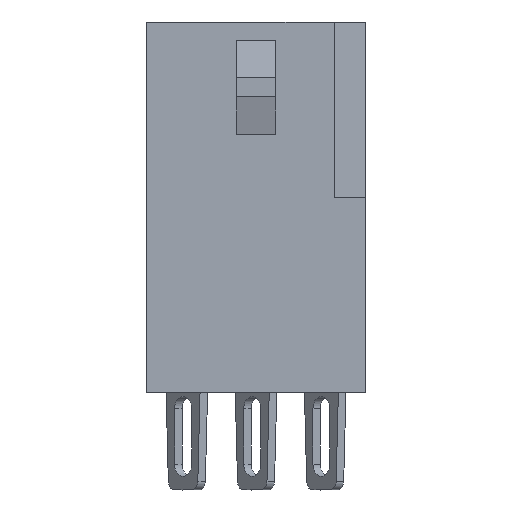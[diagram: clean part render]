
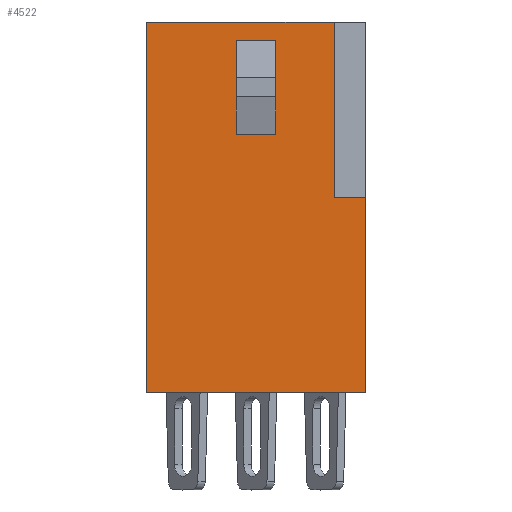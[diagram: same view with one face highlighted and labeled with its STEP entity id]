
A CAD part, top view. The second image highlights one B-rep face of the part: STEP entity #4522.
In plain terms, the highlighted planar face has unit normal (0, 0, 1).
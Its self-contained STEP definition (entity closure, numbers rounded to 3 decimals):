
#67 = EDGE_CURVE ( 'NONE', #673, #4810, #5719, .T. ) ;
#171 = LINE ( 'NONE', #1245, #2292 ) ;
#212 = CARTESIAN_POINT ( 'NONE',  ( 5.105, 8.991, 2.54 ) ) ;
#355 = CARTESIAN_POINT ( 'NONE',  ( 5.105, 8.992, 2.54 ) ) ;
#487 = ORIENTED_EDGE ( 'NONE', *, *, #4696, .T. ) ;
#583 = LINE ( 'NONE', #5169, #4838 ) ;
#605 = LINE ( 'NONE', #882, #5481 ) ;
#640 = ORIENTED_EDGE ( 'NONE', *, *, #2614, .F. ) ;
#652 = DIRECTION ( 'NONE',  ( 0., -1., 0. ) ) ;
#673 = VERTEX_POINT ( 'NONE', #4118 ) ;
#882 = CARTESIAN_POINT ( 'NONE',  ( -2.324, 10.033, 2.54 ) ) ;
#1026 = DIRECTION ( 'NONE',  ( -1., 0., 0. ) ) ;
#1198 = DIRECTION ( 'NONE',  ( -1., 0., 0. ) ) ;
#1245 = CARTESIAN_POINT ( 'NONE',  ( 7.339, 8.991, 2.54 ) ) ;
#1329 = CARTESIAN_POINT ( 'NONE',  ( 5.105, 3.608, 2.54 ) ) ;
#1357 = EDGE_CURVE ( 'NONE', #5795, #673, #6116, .T. ) ;
#1417 = LINE ( 'NONE', #4342, #2346 ) ;
#1470 = ORIENTED_EDGE ( 'NONE', *, *, #4973, .F. ) ;
#1475 = DIRECTION ( 'NONE',  ( 0., -1., 0. ) ) ;
#1613 = CARTESIAN_POINT ( 'NONE',  ( 8.445, 10.033, 2.54 ) ) ;
#1669 = VECTOR ( 'NONE', #5410, 1000. ) ;
#1874 = EDGE_CURVE ( 'NONE', #5945, #5450, #4713, .T. ) ;
#1972 = EDGE_CURVE ( 'NONE', #5797, #5795, #605, .T. ) ;
#2006 = CARTESIAN_POINT ( 'NONE',  ( -2.324, 0., 2.54 ) ) ;
#2188 = EDGE_CURVE ( 'NONE', #5945, #6157, #3814, .T. ) ;
#2202 = VERTEX_POINT ( 'NONE', #5382 ) ;
#2204 = DIRECTION ( 'NONE',  ( 1., 0., 0. ) ) ;
#2280 = VECTOR ( 'NONE', #5660, 1000. ) ;
#2292 = VECTOR ( 'NONE', #1198, 1000. ) ;
#2303 = DIRECTION ( 'NONE',  ( 1., 0., 0. ) ) ;
#2346 = VECTOR ( 'NONE', #5316, 1000. ) ;
#2416 = EDGE_CURVE ( 'NONE', #2202, #5797, #5778, .T. ) ;
#2473 = CARTESIAN_POINT ( 'NONE',  ( 8.445, 44.802, 2.54 ) ) ;
#2512 = LINE ( 'NONE', #4033, #4705 ) ;
#2595 = EDGE_LOOP ( 'NONE', ( #5480, #3376, #4501, #3917, #6083, #487 ) ) ;
#2614 = EDGE_CURVE ( 'NONE', #5559, #6157, #2512, .T. ) ;
#2905 = ORIENTED_EDGE ( 'NONE', *, *, #1874, .F. ) ;
#3146 = DIRECTION ( 'NONE',  ( 0., 1., 0. ) ) ;
#3185 = VECTOR ( 'NONE', #3146, 1000. ) ;
#3228 = CARTESIAN_POINT ( 'NONE',  ( -2.324, -11.176, 2.54 ) ) ;
#3232 = DIRECTION ( 'NONE',  ( 0., 0., 1. ) ) ;
#3376 = ORIENTED_EDGE ( 'NONE', *, *, #1357, .F. ) ;
#3644 = CARTESIAN_POINT ( 'NONE',  ( 2.819, 8.991, 2.54 ) ) ;
#3814 = LINE ( 'NONE', #5430, #6220 ) ;
#3917 = ORIENTED_EDGE ( 'NONE', *, *, #2416, .F. ) ;
#3947 = CARTESIAN_POINT ( 'NONE',  ( 2.819, 3.608, 2.54 ) ) ;
#4033 = CARTESIAN_POINT ( 'NONE',  ( 2.819, 8.992, 2.54 ) ) ;
#4106 = CARTESIAN_POINT ( 'NONE',  ( -2.324, 10.033, 2.54 ) ) ;
#4118 = CARTESIAN_POINT ( 'NONE',  ( 8.445, 0., 2.54 ) ) ;
#4155 = FACE_BOUND ( 'NONE', #4716, .T. ) ;
#4281 = DIRECTION ( 'NONE',  ( 1., 0., 0. ) ) ;
#4342 = CARTESIAN_POINT ( 'NONE',  ( 10.249, -11.176, 2.54 ) ) ;
#4501 = ORIENTED_EDGE ( 'NONE', *, *, #1972, .F. ) ;
#4522 = ADVANCED_FACE ( 'NONE', ( #4155, #6207 ), #5212, .T. ) ;
#4696 = EDGE_CURVE ( 'NONE', #4813, #4810, #1417, .T. ) ;
#4705 = VECTOR ( 'NONE', #652, 1000. ) ;
#4713 = LINE ( 'NONE', #355, #2280 ) ;
#4716 = EDGE_LOOP ( 'NONE', ( #4812, #640, #1470, #2905 ) ) ;
#4810 = VERTEX_POINT ( 'NONE', #5905 ) ;
#4812 = ORIENTED_EDGE ( 'NONE', *, *, #2188, .T. ) ;
#4813 = VERTEX_POINT ( 'NONE', #5400 ) ;
#4838 = VECTOR ( 'NONE', #2303, 1000. ) ;
#4973 = EDGE_CURVE ( 'NONE', #5450, #5559, #171, .T. ) ;
#5169 = CARTESIAN_POINT ( 'NONE',  ( -2.324, -11.176, 2.54 ) ) ;
#5212 = PLANE ( 'NONE',  #5812 ) ;
#5316 = DIRECTION ( 'NONE',  ( 0., 1., 0. ) ) ;
#5382 = CARTESIAN_POINT ( 'NONE',  ( -2.324, -11.176, 2.54 ) ) ;
#5400 = CARTESIAN_POINT ( 'NONE',  ( 10.249, -11.176, 2.54 ) ) ;
#5410 = DIRECTION ( 'NONE',  ( 1., 0., 0. ) ) ;
#5430 = CARTESIAN_POINT ( 'NONE',  ( 7.339, 3.608, 2.54 ) ) ;
#5450 = VERTEX_POINT ( 'NONE', #212 ) ;
#5480 = ORIENTED_EDGE ( 'NONE', *, *, #67, .F. ) ;
#5481 = VECTOR ( 'NONE', #4281, 1000. ) ;
#5559 = VERTEX_POINT ( 'NONE', #3644 ) ;
#5586 = VECTOR ( 'NONE', #1475, 1000. ) ;
#5657 = CARTESIAN_POINT ( 'NONE',  ( -2.324, -11.176, 2.54 ) ) ;
#5660 = DIRECTION ( 'NONE',  ( 0., 1., 0. ) ) ;
#5719 = LINE ( 'NONE', #2006, #1669 ) ;
#5778 = LINE ( 'NONE', #3228, #3185 ) ;
#5795 = VERTEX_POINT ( 'NONE', #1613 ) ;
#5797 = VERTEX_POINT ( 'NONE', #4106 ) ;
#5812 = AXIS2_PLACEMENT_3D ( 'NONE', #5657, #3232, #2204 ) ;
#5905 = CARTESIAN_POINT ( 'NONE',  ( 10.249, 0., 2.54 ) ) ;
#5945 = VERTEX_POINT ( 'NONE', #1329 ) ;
#6083 = ORIENTED_EDGE ( 'NONE', *, *, #6272, .T. ) ;
#6116 = LINE ( 'NONE', #2473, #5586 ) ;
#6157 = VERTEX_POINT ( 'NONE', #3947 ) ;
#6207 = FACE_OUTER_BOUND ( 'NONE', #2595, .T. ) ;
#6220 = VECTOR ( 'NONE', #1026, 1000. ) ;
#6272 = EDGE_CURVE ( 'NONE', #2202, #4813, #583, .T. ) ;
